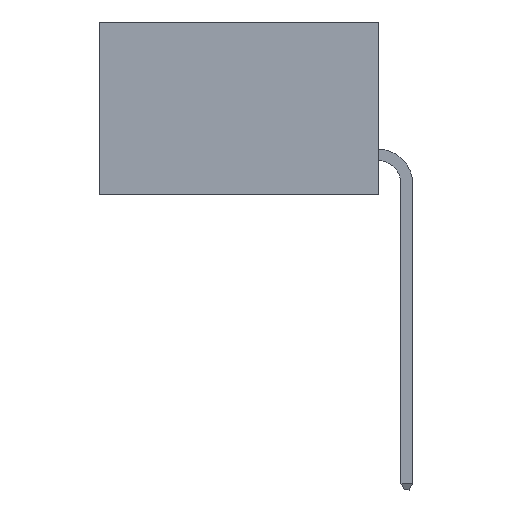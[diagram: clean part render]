
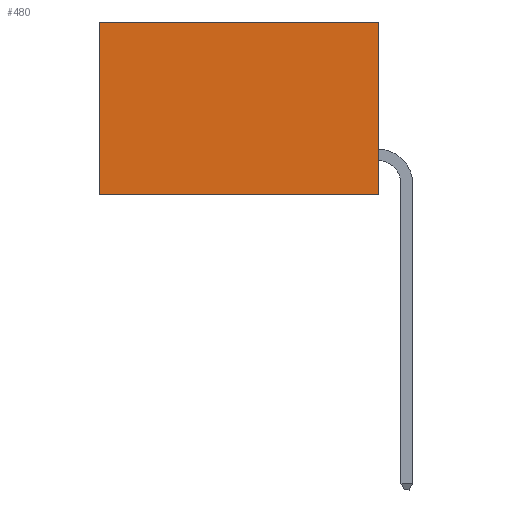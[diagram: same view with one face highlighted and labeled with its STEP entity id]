
A CAD part, left-side view. The second image highlights one B-rep face of the part: STEP entity #480.
In plain terms, the highlighted planar face has unit normal (-1, 0, 0).
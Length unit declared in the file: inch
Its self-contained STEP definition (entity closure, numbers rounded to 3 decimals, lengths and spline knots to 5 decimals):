
#184 = LINE ( 'NONE', #18481, #15222 ) ;
#480 = ADVANCED_FACE ( 'NONE', ( #14614 ), #18878, .F. ) ;
#578 = ORIENTED_EDGE ( 'NONE', *, *, #2875, .F. ) ;
#893 = CARTESIAN_POINT ( 'NONE',  ( 0.298, 0., 0. ) ) ;
#2318 = EDGE_CURVE ( 'NONE', #7182, #12388, #13432, .T. ) ;
#2808 = ORIENTED_EDGE ( 'NONE', *, *, #2318, .T. ) ;
#2875 = EDGE_CURVE ( 'NONE', #8643, #12388, #15488, .T. ) ;
#3019 = LINE ( 'NONE', #893, #13967 ) ;
#3549 = EDGE_CURVE ( 'NONE', #3757, #7182, #184, .T. ) ;
#3637 = VECTOR ( 'NONE', #7671, 39.37008 ) ;
#3757 = VERTEX_POINT ( 'NONE', #13155 ) ;
#4416 = DIRECTION ( 'NONE',  ( 0., 0., -1. ) ) ;
#6100 = ORIENTED_EDGE ( 'NONE', *, *, #14311, .F. ) ;
#6105 = EDGE_LOOP ( 'NONE', ( #2808, #578, #6100, #8140 ) ) ;
#6478 = CARTESIAN_POINT ( 'NONE',  ( 0.298, 0.6, 0. ) ) ;
#7182 = VERTEX_POINT ( 'NONE', #10780 ) ;
#7671 = DIRECTION ( 'NONE',  ( 0., 1., 0. ) ) ;
#8086 = CARTESIAN_POINT ( 'NONE',  ( 0.298, 0., -0.37 ) ) ;
#8140 = ORIENTED_EDGE ( 'NONE', *, *, #3549, .T. ) ;
#8643 = VERTEX_POINT ( 'NONE', #8086 ) ;
#9506 = VECTOR ( 'NONE', #17790, 39.37008 ) ;
#10554 = AXIS2_PLACEMENT_3D ( 'NONE', #14516, #17026, #4416 ) ;
#10780 = CARTESIAN_POINT ( 'NONE',  ( 0.298, 0.6, 0. ) ) ;
#12388 = VERTEX_POINT ( 'NONE', #17142 ) ;
#13155 = CARTESIAN_POINT ( 'NONE',  ( 0.298, 0., 0. ) ) ;
#13432 = LINE ( 'NONE', #6478, #9506 ) ;
#13967 = VECTOR ( 'NONE', #17332, 39.37008 ) ;
#14311 = EDGE_CURVE ( 'NONE', #3757, #8643, #3019, .T. ) ;
#14516 = CARTESIAN_POINT ( 'NONE',  ( 0.298, 0., 0. ) ) ;
#14614 = FACE_OUTER_BOUND ( 'NONE', #6105, .T. ) ;
#15222 = VECTOR ( 'NONE', #16818, 39.37008 ) ;
#15488 = LINE ( 'NONE', #17114, #3637 ) ;
#16818 = DIRECTION ( 'NONE',  ( 0., 1., 0. ) ) ;
#17026 = DIRECTION ( 'NONE',  ( 1., 0., 0. ) ) ;
#17114 = CARTESIAN_POINT ( 'NONE',  ( 0.298, 0., -0.37 ) ) ;
#17142 = CARTESIAN_POINT ( 'NONE',  ( 0.298, 0.6, -0.37 ) ) ;
#17332 = DIRECTION ( 'NONE',  ( 0., 0., -1. ) ) ;
#17790 = DIRECTION ( 'NONE',  ( 0., 0., -1. ) ) ;
#18481 = CARTESIAN_POINT ( 'NONE',  ( 0.298, 0., 0. ) ) ;
#18878 = PLANE ( 'NONE',  #10554 ) ;
